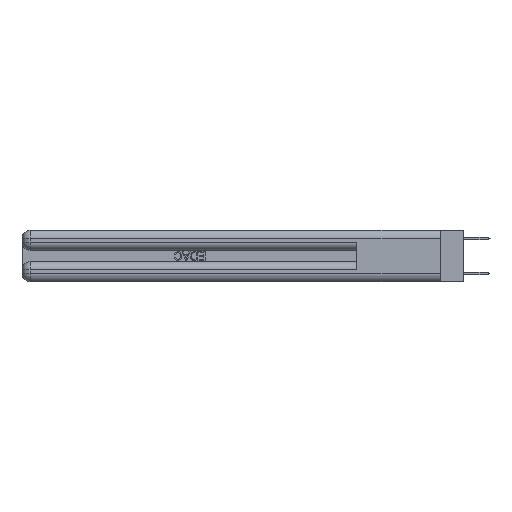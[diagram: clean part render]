
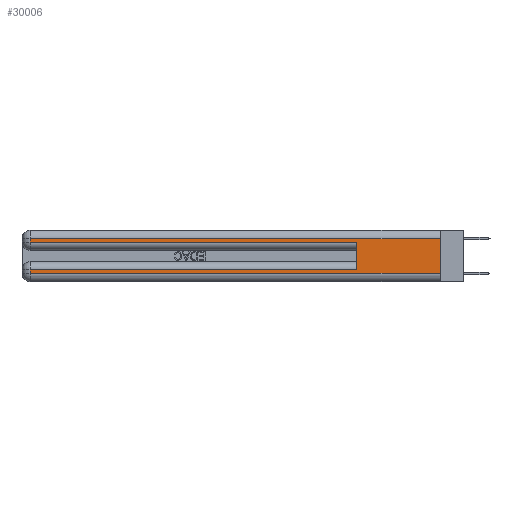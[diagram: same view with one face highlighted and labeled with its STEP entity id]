
A CAD part, left-side view. The second image highlights one B-rep face of the part: STEP entity #30006.
In plain terms, the highlighted planar face has unit normal (-1, 0, 0).
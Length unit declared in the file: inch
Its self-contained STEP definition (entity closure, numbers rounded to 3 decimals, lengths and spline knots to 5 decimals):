
#617 = CARTESIAN_POINT ( 'NONE',  ( 0., 2.94, 0.06 ) ) ;
#746 = EDGE_CURVE ( 'NONE', #14047, #2940, #16445, .T. ) ;
#2073 = DIRECTION ( 'NONE',  ( 0., 0., -1. ) ) ;
#2131 = VERTEX_POINT ( 'NONE', #23461 ) ;
#2523 = DIRECTION ( 'NONE',  ( 0., 0., 1. ) ) ;
#2551 = CARTESIAN_POINT ( 'NONE',  ( 0., 2.94, 0.285 ) ) ;
#2940 = VERTEX_POINT ( 'NONE', #2551 ) ;
#3006 = CARTESIAN_POINT ( 'NONE',  ( 0., 0., 0.285 ) ) ;
#3614 = CARTESIAN_POINT ( 'NONE',  ( 0., 2.94, 0.31 ) ) ;
#3936 = AXIS2_PLACEMENT_3D ( 'NONE', #11938, #30630, #14656 ) ;
#4089 = DIRECTION ( 'NONE',  ( 0., 0., -1. ) ) ;
#4097 = CARTESIAN_POINT ( 'NONE',  ( 0., 0., 0.31 ) ) ;
#4245 = CARTESIAN_POINT ( 'NONE',  ( 0., 2.94, 0.37 ) ) ;
#4542 = EDGE_LOOP ( 'NONE', ( #23945, #5061, #34926, #33316, #14901, #5725, #21788, #19243 ) ) ;
#4950 = LINE ( 'NONE', #21128, #12234 ) ;
#5061 = ORIENTED_EDGE ( 'NONE', *, *, #8210, .T. ) ;
#5725 = ORIENTED_EDGE ( 'NONE', *, *, #23323, .T. ) ;
#7388 = VERTEX_POINT ( 'NONE', #617 ) ;
#7654 = VECTOR ( 'NONE', #33610, 39.37008 ) ;
#8165 = LINE ( 'NONE', #21549, #20007 ) ;
#8210 = EDGE_CURVE ( 'NONE', #12573, #14047, #21183, .T. ) ;
#8320 = DIRECTION ( 'NONE',  ( 0., -1., 0. ) ) ;
#10045 = EDGE_CURVE ( 'NONE', #12573, #11804, #32268, .T. ) ;
#10084 = VECTOR ( 'NONE', #4089, 39.37008 ) ;
#11455 = CARTESIAN_POINT ( 'NONE',  ( 0., 0., 0.06 ) ) ;
#11795 = VECTOR ( 'NONE', #33112, 39.37008 ) ;
#11804 = VERTEX_POINT ( 'NONE', #11455 ) ;
#11855 = LINE ( 'NONE', #32325, #32331 ) ;
#11938 = CARTESIAN_POINT ( 'NONE',  ( 0., 0., 0.37 ) ) ;
#12234 = VECTOR ( 'NONE', #2073, 39.37008 ) ;
#12573 = VERTEX_POINT ( 'NONE', #26999 ) ;
#13998 = VERTEX_POINT ( 'NONE', #14439 ) ;
#14047 = VERTEX_POINT ( 'NONE', #3614 ) ;
#14439 = CARTESIAN_POINT ( 'NONE',  ( 0., 0.6, 0.285 ) ) ;
#14639 = LINE ( 'NONE', #31686, #29654 ) ;
#14656 = DIRECTION ( 'NONE',  ( 0., 0., -1. ) ) ;
#14901 = ORIENTED_EDGE ( 'NONE', *, *, #30443, .F. ) ;
#15763 = DIRECTION ( 'NONE',  ( 0., 1., 0. ) ) ;
#16445 = LINE ( 'NONE', #4245, #10084 ) ;
#16633 = CARTESIAN_POINT ( 'NONE',  ( 0., 0.6, 0.085 ) ) ;
#19243 = ORIENTED_EDGE ( 'NONE', *, *, #19771, .T. ) ;
#19771 = EDGE_CURVE ( 'NONE', #7388, #11804, #11855, .T. ) ;
#20007 = VECTOR ( 'NONE', #2523, 39.37008 ) ;
#21128 = CARTESIAN_POINT ( 'NONE',  ( 0., 2.94, 0.37 ) ) ;
#21183 = LINE ( 'NONE', #4097, #7654 ) ;
#21543 = EDGE_CURVE ( 'NONE', #2131, #7388, #4950, .T. ) ;
#21549 = CARTESIAN_POINT ( 'NONE',  ( 0., 0.6, 0.145 ) ) ;
#21788 = ORIENTED_EDGE ( 'NONE', *, *, #21543, .T. ) ;
#22016 = DIRECTION ( 'NONE',  ( 0., -1., 0. ) ) ;
#23323 = EDGE_CURVE ( 'NONE', #33330, #2131, #14639, .T. ) ;
#23461 = CARTESIAN_POINT ( 'NONE',  ( 0., 2.94, 0.085 ) ) ;
#23945 = ORIENTED_EDGE ( 'NONE', *, *, #10045, .F. ) ;
#26926 = LINE ( 'NONE', #3006, #33975 ) ;
#26999 = CARTESIAN_POINT ( 'NONE',  ( 0., 0., 0.31 ) ) ;
#27927 = PLANE ( 'NONE',  #3936 ) ;
#29654 = VECTOR ( 'NONE', #15763, 39.37008 ) ;
#30006 = ADVANCED_FACE ( 'NONE', ( #33296 ), #27927, .F. ) ;
#30443 = EDGE_CURVE ( 'NONE', #33330, #13998, #8165, .T. ) ;
#30468 = CARTESIAN_POINT ( 'NONE',  ( 0., 0., 0.37 ) ) ;
#30630 = DIRECTION ( 'NONE',  ( 1., 0., 0. ) ) ;
#31686 = CARTESIAN_POINT ( 'NONE',  ( 0., 0., 0.085 ) ) ;
#32219 = EDGE_CURVE ( 'NONE', #2940, #13998, #26926, .T. ) ;
#32268 = LINE ( 'NONE', #30468, #11795 ) ;
#32325 = CARTESIAN_POINT ( 'NONE',  ( 0., 0., 0.06 ) ) ;
#32331 = VECTOR ( 'NONE', #8320, 39.37008 ) ;
#33112 = DIRECTION ( 'NONE',  ( 0., 0., -1. ) ) ;
#33296 = FACE_OUTER_BOUND ( 'NONE', #4542, .T. ) ;
#33316 = ORIENTED_EDGE ( 'NONE', *, *, #32219, .T. ) ;
#33330 = VERTEX_POINT ( 'NONE', #16633 ) ;
#33610 = DIRECTION ( 'NONE',  ( 0., 1., 0. ) ) ;
#33975 = VECTOR ( 'NONE', #22016, 39.37008 ) ;
#34926 = ORIENTED_EDGE ( 'NONE', *, *, #746, .T. ) ;
